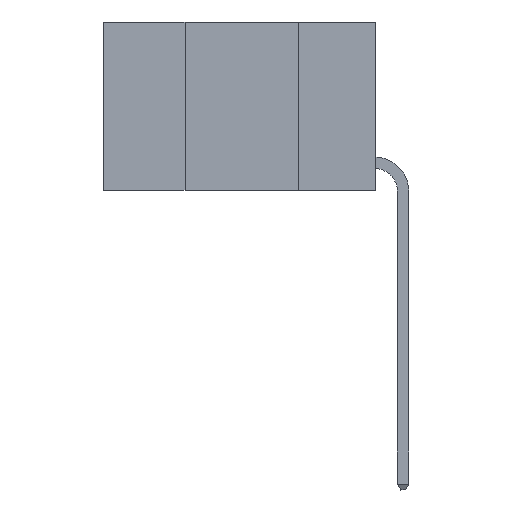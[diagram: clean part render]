
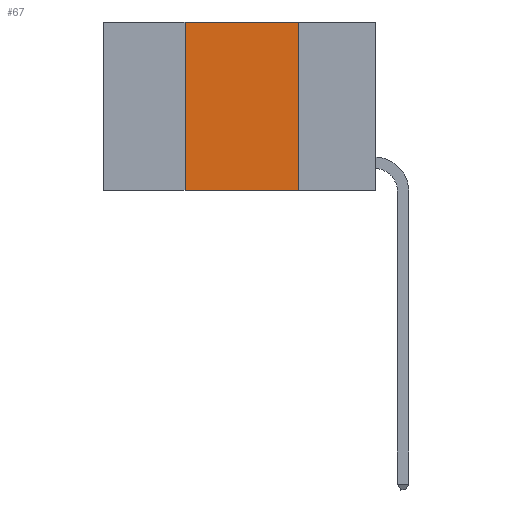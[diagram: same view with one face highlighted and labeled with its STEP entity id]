
A CAD part, left-side view. The second image highlights one B-rep face of the part: STEP entity #67.
In plain terms, the highlighted planar face has unit normal (-1, 0, 0).
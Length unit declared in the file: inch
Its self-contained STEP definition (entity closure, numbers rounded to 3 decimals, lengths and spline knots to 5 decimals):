
#67 = ADVANCED_FACE ( 'NONE', ( #5705 ), #4128, .F. ) ;
#223 = CARTESIAN_POINT ( 'NONE',  ( 0., 0.6, -0.37 ) ) ;
#491 = CARTESIAN_POINT ( 'NONE',  ( 0., 0.17, 0. ) ) ;
#994 = VECTOR ( 'NONE', #7581, 39.37008 ) ;
#1951 = CARTESIAN_POINT ( 'NONE',  ( 0., 0.17, -0.37 ) ) ;
#2053 = DIRECTION ( 'NONE',  ( 0., -1., 0. ) ) ;
#2066 = ORIENTED_EDGE ( 'NONE', *, *, #12957, .T. ) ;
#2227 = CARTESIAN_POINT ( 'NONE',  ( 0., 0.42, -0.37 ) ) ;
#2700 = CARTESIAN_POINT ( 'NONE',  ( 0., 0.42, 0. ) ) ;
#3717 = DIRECTION ( 'NONE',  ( 0., 0., -1. ) ) ;
#4128 = PLANE ( 'NONE',  #13976 ) ;
#5705 = FACE_OUTER_BOUND ( 'NONE', #12201, .T. ) ;
#6469 = EDGE_CURVE ( 'NONE', #14002, #6780, #12373, .T. ) ;
#6780 = VERTEX_POINT ( 'NONE', #2700 ) ;
#6817 = VECTOR ( 'NONE', #11392, 39.37008 ) ;
#7581 = DIRECTION ( 'NONE',  ( 0., 0., 1. ) ) ;
#8030 = ORIENTED_EDGE ( 'NONE', *, *, #6469, .F. ) ;
#8803 = VERTEX_POINT ( 'NONE', #1951 ) ;
#8846 = DIRECTION ( 'NONE',  ( 0., 0., -1. ) ) ;
#8931 = EDGE_CURVE ( 'NONE', #6780, #14869, #19840, .T. ) ;
#10149 = ORIENTED_EDGE ( 'NONE', *, *, #14773, .F. ) ;
#10606 = CARTESIAN_POINT ( 'NONE',  ( 0., 0.42, 0. ) ) ;
#10615 = CARTESIAN_POINT ( 'NONE',  ( 0., 0.17, 0. ) ) ;
#11392 = DIRECTION ( 'NONE',  ( 0., -1., 0. ) ) ;
#12011 = VECTOR ( 'NONE', #2053, 39.37008 ) ;
#12201 = EDGE_LOOP ( 'NONE', ( #10149, #18403, #8030, #2066 ) ) ;
#12373 = LINE ( 'NONE', #10606, #994 ) ;
#12957 = EDGE_CURVE ( 'NONE', #14002, #8803, #14538, .T. ) ;
#13855 = DIRECTION ( 'NONE',  ( 1., 0., 0. ) ) ;
#13976 = AXIS2_PLACEMENT_3D ( 'NONE', #17212, #13855, #8846 ) ;
#14002 = VERTEX_POINT ( 'NONE', #2227 ) ;
#14538 = LINE ( 'NONE', #223, #6817 ) ;
#14773 = EDGE_CURVE ( 'NONE', #14869, #8803, #14819, .T. ) ;
#14819 = LINE ( 'NONE', #491, #18852 ) ;
#14869 = VERTEX_POINT ( 'NONE', #10615 ) ;
#17212 = CARTESIAN_POINT ( 'NONE',  ( 0., 0.6, 0. ) ) ;
#17964 = CARTESIAN_POINT ( 'NONE',  ( 0., 0.6, 0. ) ) ;
#18403 = ORIENTED_EDGE ( 'NONE', *, *, #8931, .F. ) ;
#18852 = VECTOR ( 'NONE', #3717, 39.37008 ) ;
#19840 = LINE ( 'NONE', #17964, #12011 ) ;
